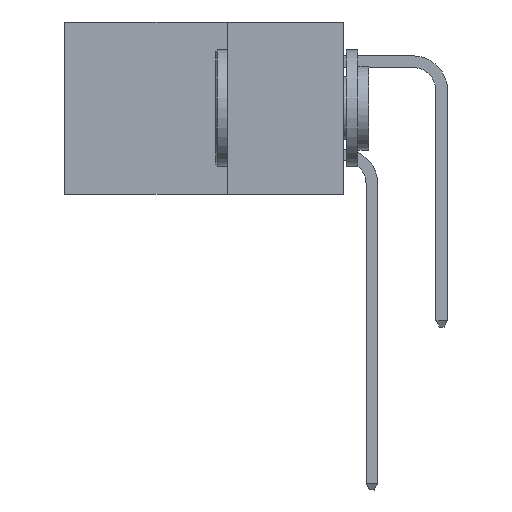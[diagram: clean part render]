
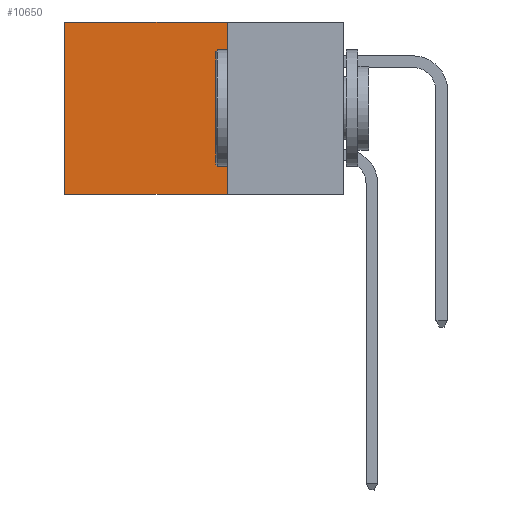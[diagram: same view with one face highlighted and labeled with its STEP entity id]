
A CAD part, left-side view. The second image highlights one B-rep face of the part: STEP entity #10650.
In plain terms, the highlighted planar face has unit normal (-1, 0, 0).
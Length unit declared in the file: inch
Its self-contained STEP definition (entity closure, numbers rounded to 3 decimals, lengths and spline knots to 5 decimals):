
#563 = EDGE_CURVE ( 'NONE', #5158, #7230, #6407, .T. ) ;
#635 = VERTEX_POINT ( 'NONE', #1771 ) ;
#717 = LINE ( 'NONE', #6271, #8835 ) ;
#1771 = CARTESIAN_POINT ( 'NONE',  ( 0.2615, 0.25, -0.37 ) ) ;
#1975 = VERTEX_POINT ( 'NONE', #8401 ) ;
#2571 = CARTESIAN_POINT ( 'NONE',  ( 0.2615, 0.25, -0.37 ) ) ;
#2852 = DIRECTION ( 'NONE',  ( 0., 1., 0. ) ) ;
#2947 = CARTESIAN_POINT ( 'NONE',  ( 0.2615, 0.25, -0.37 ) ) ;
#3211 = VECTOR ( 'NONE', #8952, 39.37008 ) ;
#3390 = DIRECTION ( 'NONE',  ( 0., 0., -1. ) ) ;
#3546 = EDGE_CURVE ( 'NONE', #5158, #635, #7877, .T. ) ;
#3976 = DIRECTION ( 'NONE',  ( 0., 0., -1. ) ) ;
#4571 = DIRECTION ( 'NONE',  ( 0., 0., -1. ) ) ;
#4729 = VECTOR ( 'NONE', #2852, 39.37008 ) ;
#4921 = CARTESIAN_POINT ( 'NONE',  ( 0.2615, 0.25, -0.37 ) ) ;
#5087 = PLANE ( 'NONE',  #10432 ) ;
#5098 = VECTOR ( 'NONE', #4571, 39.37008 ) ;
#5158 = VERTEX_POINT ( 'NONE', #10834 ) ;
#6122 = ORIENTED_EDGE ( 'NONE', *, *, #6698, .F. ) ;
#6167 = ORIENTED_EDGE ( 'NONE', *, *, #8539, .T. ) ;
#6271 = CARTESIAN_POINT ( 'NONE',  ( 0.2615, 0.6, -0.37 ) ) ;
#6283 = ORIENTED_EDGE ( 'NONE', *, *, #563, .T. ) ;
#6407 = LINE ( 'NONE', #10959, #3211 ) ;
#6698 = EDGE_CURVE ( 'NONE', #635, #1975, #7674, .T. ) ;
#7230 = VERTEX_POINT ( 'NONE', #9476 ) ;
#7674 = LINE ( 'NONE', #4921, #4729 ) ;
#7713 = DIRECTION ( 'NONE',  ( 1., 0., 0. ) ) ;
#7877 = LINE ( 'NONE', #2571, #5098 ) ;
#8401 = CARTESIAN_POINT ( 'NONE',  ( 0.2615, 0.6, -0.37 ) ) ;
#8539 = EDGE_CURVE ( 'NONE', #7230, #1975, #717, .T. ) ;
#8835 = VECTOR ( 'NONE', #3390, 39.37008 ) ;
#8952 = DIRECTION ( 'NONE',  ( 0., 1., 0. ) ) ;
#9476 = CARTESIAN_POINT ( 'NONE',  ( 0.2615, 0.6, 0. ) ) ;
#10432 = AXIS2_PLACEMENT_3D ( 'NONE', #2947, #7713, #3976 ) ;
#10650 = ADVANCED_FACE ( 'NONE', ( #11516 ), #5087, .F. ) ;
#10834 = CARTESIAN_POINT ( 'NONE',  ( 0.2615, 0.25, 0. ) ) ;
#10869 = ORIENTED_EDGE ( 'NONE', *, *, #3546, .F. ) ;
#10959 = CARTESIAN_POINT ( 'NONE',  ( 0.2615, 0.25, 0. ) ) ;
#11516 = FACE_OUTER_BOUND ( 'NONE', #11523, .T. ) ;
#11523 = EDGE_LOOP ( 'NONE', ( #6167, #6122, #10869, #6283 ) ) ;
